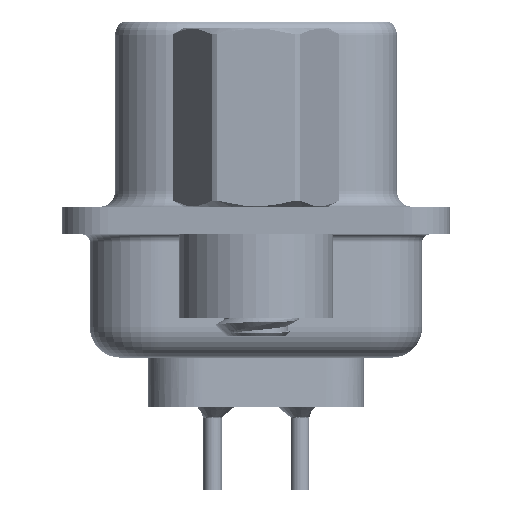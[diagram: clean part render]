
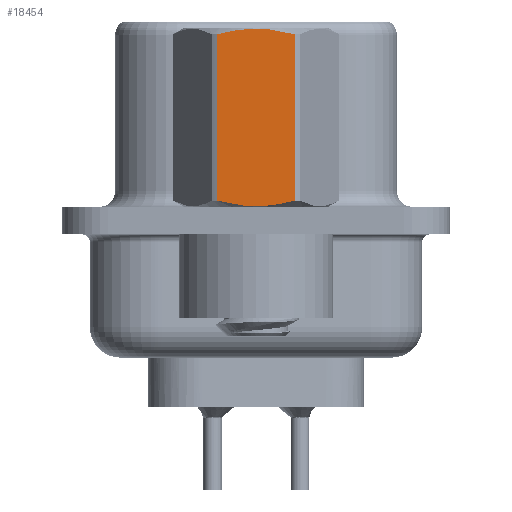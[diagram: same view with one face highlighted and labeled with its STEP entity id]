
A CAD part, left-side view. The second image highlights one B-rep face of the part: STEP entity #18454.
In plain terms, the highlighted planar face has unit normal (-1, 0, 0).
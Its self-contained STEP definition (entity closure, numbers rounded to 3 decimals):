
#996 = CARTESIAN_POINT ( 'NONE',  ( -2.381, 1.273, 3.792 ) ) ;
#1212 = DIRECTION ( 'NONE',  ( 0., 0., -1. ) ) ;
#1617 = VERTEX_POINT ( 'NONE', #19437 ) ;
#2011 = VERTEX_POINT ( 'NONE', #28247 ) ;
#2240 = EDGE_CURVE ( 'NONE', #27690, #2011, #6913, .T. ) ;
#2332 = CARTESIAN_POINT ( 'NONE',  ( -2.381, 0.215, 0.468 ) ) ;
#3927 = CARTESIAN_POINT ( 'NONE',  ( -2.381, -0.432, 6.215 ) ) ;
#4821 = VECTOR ( 'NONE', #21279, 1000. ) ;
#4879 = CARTESIAN_POINT ( 'NONE',  ( -2.381, 1.273, 6.048 ) ) ;
#4887 = CARTESIAN_POINT ( 'NONE',  ( -2.381, 1.273, 0.652 ) ) ;
#4993 = CARTESIAN_POINT ( 'NONE',  ( -2.381, -0.432, 0.485 ) ) ;
#5566 = DIRECTION ( 'NONE',  ( -1., 0., 0. ) ) ;
#5647 = LINE ( 'NONE', #34341, #4821 ) ;
#6556 = CARTESIAN_POINT ( 'NONE',  ( -2.381, 0.215, 6.232 ) ) ;
#6613 = ORIENTED_EDGE ( 'NONE', *, *, #10972, .T. ) ;
#6913 = LINE ( 'NONE', #996, #21032 ) ;
#7659 = CARTESIAN_POINT ( 'NONE',  ( -2.381, -1.066, 0.596 ) ) ;
#9243 = CARTESIAN_POINT ( 'NONE',  ( -2.381, 0.853, 6.151 ) ) ;
#10972 = EDGE_CURVE ( 'NONE', #1617, #27690, #13466, .T. ) ;
#13466 = B_SPLINE_CURVE_WITH_KNOTS ( 'NONE', 3,
 ( #32941, #14433, #19796, #3927, #22414, #6556, #25064, #9243, #31454, #26382 ),
 .UNSPECIFIED., .F., .F.,
 ( 4, 2, 2, 2, 4 ),
 ( 0.001, 0.002, 0.002, 0.003, 0.004 ),
 .UNSPECIFIED. ) ;
#14433 = CARTESIAN_POINT ( 'NONE',  ( -2.381, -1.066, 6.104 ) ) ;
#15449 = VERTEX_POINT ( 'NONE', #33111 ) ;
#15779 = FACE_OUTER_BOUND ( 'NONE', #26318, .T. ) ;
#16104 = CARTESIAN_POINT ( 'NONE',  ( -2.381, 1.375, -3.75 ) ) ;
#16130 = ORIENTED_EDGE ( 'NONE', *, *, #16860, .T. ) ;
#16860 = EDGE_CURVE ( 'NONE', #2011, #15449, #17514, .T. ) ;
#17514 = B_SPLINE_CURVE_WITH_KNOTS ( 'NONE', 3,
 ( #4887, #18090, #34046, #18207, #2332, #20866, #4993, #23501, #7659, #26142 ),
 .UNSPECIFIED., .F., .F.,
 ( 4, 2, 2, 2, 4 ),
 ( 0.003, 0.003, 0.004, 0.004, 0.005 ),
 .UNSPECIFIED. ) ;
#18090 = CARTESIAN_POINT ( 'NONE',  ( -2.381, 1.065, 0.596 ) ) ;
#18207 = CARTESIAN_POINT ( 'NONE',  ( -2.381, 0.428, 0.485 ) ) ;
#18454 = ADVANCED_FACE ( 'NONE', ( #15779 ), #21421, .T. ) ;
#19437 = CARTESIAN_POINT ( 'NONE',  ( -2.381, -1.273, 6.048 ) ) ;
#19796 = CARTESIAN_POINT ( 'NONE',  ( -2.381, -0.858, 6.15 ) ) ;
#20866 = CARTESIAN_POINT ( 'NONE',  ( -2.381, -0.215, 0.468 ) ) ;
#21032 = VECTOR ( 'NONE', #1212, 1000. ) ;
#21279 = DIRECTION ( 'NONE',  ( 0., 0., 1. ) ) ;
#21421 = PLANE ( 'NONE',  #22750 ) ;
#21951 = EDGE_CURVE ( 'NONE', #15449, #1617, #5647, .T. ) ;
#22414 = CARTESIAN_POINT ( 'NONE',  ( -2.381, -0.215, 6.232 ) ) ;
#22750 = AXIS2_PLACEMENT_3D ( 'NONE', #16104, #5566, #24075 ) ;
#23501 = CARTESIAN_POINT ( 'NONE',  ( -2.381, -0.858, 0.55 ) ) ;
#23832 = ORIENTED_EDGE ( 'NONE', *, *, #21951, .T. ) ;
#24075 = DIRECTION ( 'NONE',  ( 0., -1., 0. ) ) ;
#25064 = CARTESIAN_POINT ( 'NONE',  ( -2.381, 0.428, 6.215 ) ) ;
#26142 = CARTESIAN_POINT ( 'NONE',  ( -2.381, -1.273, 0.652 ) ) ;
#26318 = EDGE_LOOP ( 'NONE', ( #16130, #23832, #6613, #33074 ) ) ;
#26382 = CARTESIAN_POINT ( 'NONE',  ( -2.381, 1.273, 6.048 ) ) ;
#27690 = VERTEX_POINT ( 'NONE', #4879 ) ;
#28247 = CARTESIAN_POINT ( 'NONE',  ( -2.381, 1.273, 0.652 ) ) ;
#31454 = CARTESIAN_POINT ( 'NONE',  ( -2.381, 1.065, 6.104 ) ) ;
#32941 = CARTESIAN_POINT ( 'NONE',  ( -2.381, -1.273, 6.048 ) ) ;
#33074 = ORIENTED_EDGE ( 'NONE', *, *, #2240, .T. ) ;
#33111 = CARTESIAN_POINT ( 'NONE',  ( -2.381, -1.273, 0.652 ) ) ;
#34046 = CARTESIAN_POINT ( 'NONE',  ( -2.381, 0.853, 0.549 ) ) ;
#34341 = CARTESIAN_POINT ( 'NONE',  ( -2.381, -1.273, 3.792 ) ) ;
